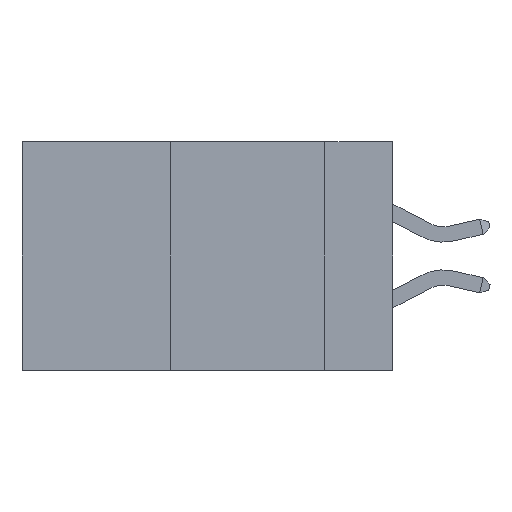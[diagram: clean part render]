
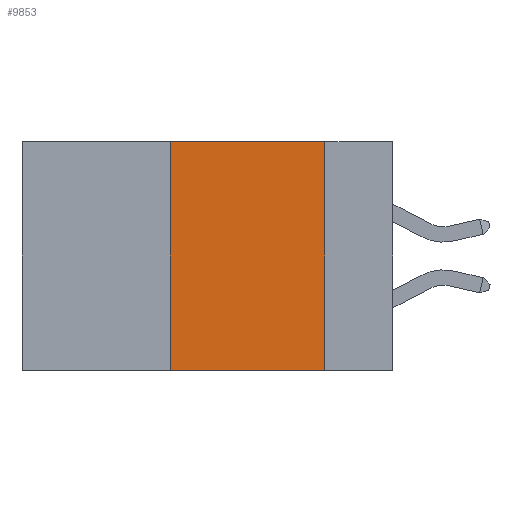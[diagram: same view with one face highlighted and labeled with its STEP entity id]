
A CAD part, left-side view. The second image highlights one B-rep face of the part: STEP entity #9853.
In plain terms, the highlighted planar face has unit normal (-1, 0, 0).
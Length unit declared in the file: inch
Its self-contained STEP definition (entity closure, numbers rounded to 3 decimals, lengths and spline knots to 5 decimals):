
#73 = CARTESIAN_POINT ( 'NONE',  ( 0., 0.11, 0. ) ) ;
#171 = DIRECTION ( 'NONE',  ( 0., 0., -1. ) ) ;
#1050 = VERTEX_POINT ( 'NONE', #14822 ) ;
#1770 = LINE ( 'NONE', #73, #2513 ) ;
#2513 = VECTOR ( 'NONE', #171, 39.37008 ) ;
#3434 = CARTESIAN_POINT ( 'NONE',  ( 0., 0.11, 0. ) ) ;
#5208 = LINE ( 'NONE', #7229, #17256 ) ;
#6516 = LINE ( 'NONE', #18792, #26515 ) ;
#6728 = EDGE_CURVE ( 'NONE', #1050, #25020, #6516, .T. ) ;
#7229 = CARTESIAN_POINT ( 'NONE',  ( 0., 0.6, 0. ) ) ;
#7461 = FACE_OUTER_BOUND ( 'NONE', #20208, .T. ) ;
#8767 = PLANE ( 'NONE',  #24420 ) ;
#9827 = ORIENTED_EDGE ( 'NONE', *, *, #27790, .F. ) ;
#9853 = ADVANCED_FACE ( 'NONE', ( #7461 ), #8767, .F. ) ;
#11205 = CARTESIAN_POINT ( 'NONE',  ( 0., 0.6, 0. ) ) ;
#12384 = ORIENTED_EDGE ( 'NONE', *, *, #16030, .F. ) ;
#12888 = CARTESIAN_POINT ( 'NONE',  ( 0., 0.36, 0. ) ) ;
#14822 = CARTESIAN_POINT ( 'NONE',  ( 0., 0.36, -0.37 ) ) ;
#15000 = DIRECTION ( 'NONE',  ( 0., 0., 1. ) ) ;
#15209 = EDGE_CURVE ( 'NONE', #22069, #28154, #5208, .T. ) ;
#15357 = VECTOR ( 'NONE', #15000, 39.37008 ) ;
#16030 = EDGE_CURVE ( 'NONE', #1050, #22069, #24789, .T. ) ;
#17256 = VECTOR ( 'NONE', #29160, 39.37008 ) ;
#17642 = CARTESIAN_POINT ( 'NONE',  ( 0., 0.36, 0. ) ) ;
#18792 = CARTESIAN_POINT ( 'NONE',  ( 0., 0.6, -0.37 ) ) ;
#20208 = EDGE_LOOP ( 'NONE', ( #9827, #26812, #12384, #22511 ) ) ;
#22069 = VERTEX_POINT ( 'NONE', #17642 ) ;
#22511 = ORIENTED_EDGE ( 'NONE', *, *, #6728, .T. ) ;
#24420 = AXIS2_PLACEMENT_3D ( 'NONE', #11205, #28187, #28083 ) ;
#24789 = LINE ( 'NONE', #12888, #15357 ) ;
#25020 = VERTEX_POINT ( 'NONE', #30321 ) ;
#26515 = VECTOR ( 'NONE', #30532, 39.37008 ) ;
#26812 = ORIENTED_EDGE ( 'NONE', *, *, #15209, .F. ) ;
#27790 = EDGE_CURVE ( 'NONE', #28154, #25020, #1770, .T. ) ;
#28083 = DIRECTION ( 'NONE',  ( 0., 0., -1. ) ) ;
#28154 = VERTEX_POINT ( 'NONE', #3434 ) ;
#28187 = DIRECTION ( 'NONE',  ( 1., 0., 0. ) ) ;
#29160 = DIRECTION ( 'NONE',  ( 0., -1., 0. ) ) ;
#30321 = CARTESIAN_POINT ( 'NONE',  ( 0., 0.11, -0.37 ) ) ;
#30532 = DIRECTION ( 'NONE',  ( 0., -1., 0. ) ) ;
